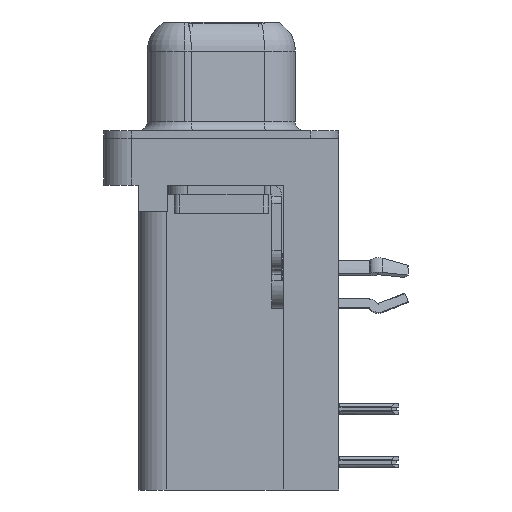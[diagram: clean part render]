
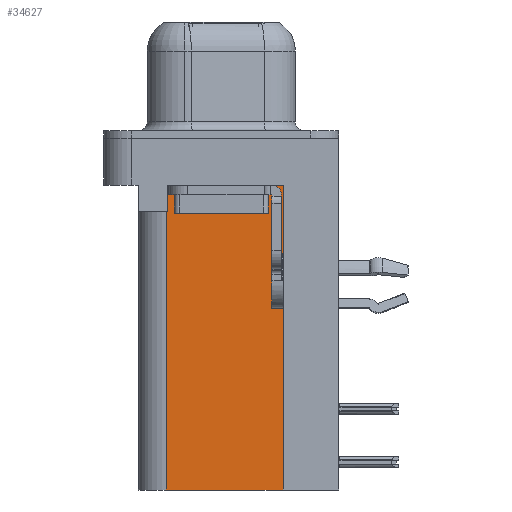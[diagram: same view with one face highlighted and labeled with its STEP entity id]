
A CAD part, left-side view. The second image highlights one B-rep face of the part: STEP entity #34627.
In plain terms, the highlighted planar face has unit normal (-1, 0, 0).
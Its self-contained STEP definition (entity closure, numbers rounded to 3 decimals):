
#315 = DIRECTION ( 'NONE',  ( 1., 0., 0. ) ) ;
#508 = CARTESIAN_POINT ( 'NONE',  ( 3.79, 2.925, -18.76 ) ) ;
#1821 = CARTESIAN_POINT ( 'NONE',  ( 3.79, 2.895, -2.5 ) ) ;
#2471 = VECTOR ( 'NONE', #26473, 1000. ) ;
#2639 = CARTESIAN_POINT ( 'NONE',  ( 3.79, 2.895, -3.9 ) ) ;
#3267 = LINE ( 'NONE', #35445, #2471 ) ;
#4094 = FACE_OUTER_BOUND ( 'NONE', #14848, .T. ) ;
#4649 = LINE ( 'NONE', #32185, #5039 ) ;
#5039 = VECTOR ( 'NONE', #35152, 1000. ) ;
#6500 = VERTEX_POINT ( 'NONE', #11172 ) ;
#7696 = VECTOR ( 'NONE', #11552, 1000. ) ;
#7927 = LINE ( 'NONE', #32502, #7696 ) ;
#9234 = EDGE_CURVE ( 'NONE', #16909, #15020, #4649, .T. ) ;
#9589 = CARTESIAN_POINT ( 'NONE',  ( 3.79, -3.295, -18.76 ) ) ;
#11172 = CARTESIAN_POINT ( 'NONE',  ( 3.79, -3.295, -18.76 ) ) ;
#11552 = DIRECTION ( 'NONE',  ( 0., 1., 0. ) ) ;
#11657 = EDGE_CURVE ( 'NONE', #6500, #16909, #27070, .T. ) ;
#12188 = EDGE_CURVE ( 'NONE', #6500, #31734, #23463, .T. ) ;
#14848 = EDGE_LOOP ( 'NONE', ( #32476, #29961, #35495, #20695, #35765, #35148 ) ) ;
#15020 = VERTEX_POINT ( 'NONE', #17710 ) ;
#16521 = VERTEX_POINT ( 'NONE', #1821 ) ;
#16909 = VERTEX_POINT ( 'NONE', #508 ) ;
#17710 = CARTESIAN_POINT ( 'NONE',  ( 3.79, 2.925, -3.9 ) ) ;
#18610 = CARTESIAN_POINT ( 'NONE',  ( 3.79, -3.295, -2.5 ) ) ;
#20286 = EDGE_CURVE ( 'NONE', #31734, #16521, #3267, .T. ) ;
#20695 = ORIENTED_EDGE ( 'NONE', *, *, #9234, .F. ) ;
#20771 = DIRECTION ( 'NONE',  ( 0., 1., 0. ) ) ;
#23101 = DIRECTION ( 'NONE',  ( 0., 0., -1. ) ) ;
#23262 = VECTOR ( 'NONE', #31574, 1000. ) ;
#23463 = LINE ( 'NONE', #28530, #23262 ) ;
#24336 = DIRECTION ( 'NONE',  ( 0., 1., 0. ) ) ;
#26160 = AXIS2_PLACEMENT_3D ( 'NONE', #32762, #315, #20771 ) ;
#26473 = DIRECTION ( 'NONE',  ( 0., 1., 0. ) ) ;
#26901 = VECTOR ( 'NONE', #24336, 1000. ) ;
#27070 = LINE ( 'NONE', #9589, #26901 ) ;
#28530 = CARTESIAN_POINT ( 'NONE',  ( 3.79, -3.295, -18.76 ) ) ;
#29961 = ORIENTED_EDGE ( 'NONE', *, *, #35666, .T. ) ;
#31574 = DIRECTION ( 'NONE',  ( 0., 0., 1. ) ) ;
#31734 = VERTEX_POINT ( 'NONE', #18610 ) ;
#32185 = CARTESIAN_POINT ( 'NONE',  ( 3.79, 2.925, -18.76 ) ) ;
#32476 = ORIENTED_EDGE ( 'NONE', *, *, #20286, .T. ) ;
#32502 = CARTESIAN_POINT ( 'NONE',  ( 3.79, 0., -3.9 ) ) ;
#32762 = CARTESIAN_POINT ( 'NONE',  ( 3.79, -3.295, -18.76 ) ) ;
#33650 = CARTESIAN_POINT ( 'NONE',  ( 3.79, 2.895, -3.9 ) ) ;
#33956 = EDGE_CURVE ( 'NONE', #34824, #15020, #7927, .T. ) ;
#34627 = ADVANCED_FACE ( 'NONE', ( #4094 ), #35677, .F. ) ;
#34824 = VERTEX_POINT ( 'NONE', #33650 ) ;
#35148 = ORIENTED_EDGE ( 'NONE', *, *, #12188, .T. ) ;
#35152 = DIRECTION ( 'NONE',  ( 0., 0., 1. ) ) ;
#35335 = LINE ( 'NONE', #2639, #35460 ) ;
#35445 = CARTESIAN_POINT ( 'NONE',  ( 3.79, -3.295, -2.5 ) ) ;
#35460 = VECTOR ( 'NONE', #23101, 1000. ) ;
#35495 = ORIENTED_EDGE ( 'NONE', *, *, #33956, .T. ) ;
#35666 = EDGE_CURVE ( 'NONE', #16521, #34824, #35335, .T. ) ;
#35677 = PLANE ( 'NONE',  #26160 ) ;
#35765 = ORIENTED_EDGE ( 'NONE', *, *, #11657, .F. ) ;
